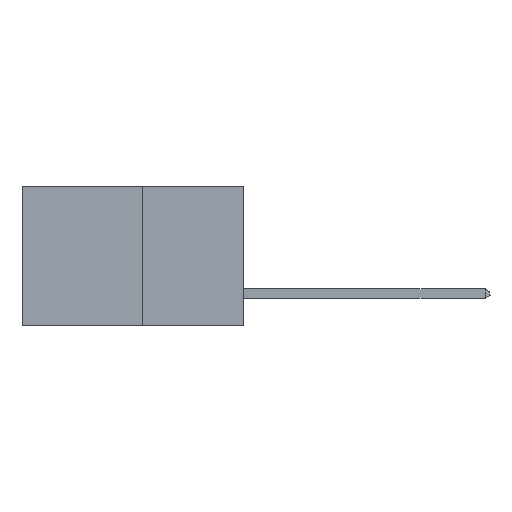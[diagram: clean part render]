
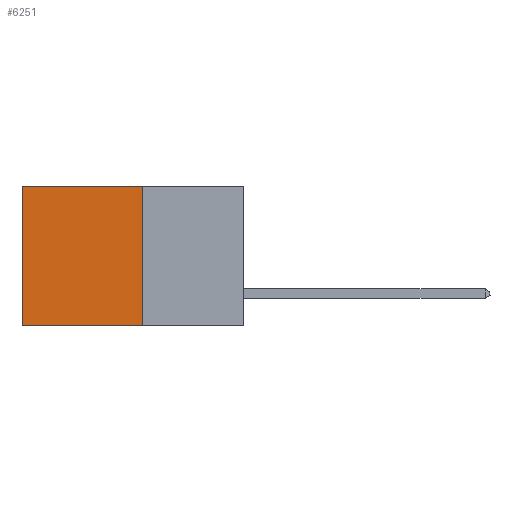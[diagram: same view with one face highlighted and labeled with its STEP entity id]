
A CAD part, left-side view. The second image highlights one B-rep face of the part: STEP entity #6251.
In plain terms, the highlighted planar face has unit normal (-1, 0, 0).
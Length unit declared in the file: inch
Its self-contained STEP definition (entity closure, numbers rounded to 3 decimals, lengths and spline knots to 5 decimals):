
#93 = DIRECTION ( 'NONE',  ( 0., 1., 0. ) ) ;
#866 = ORIENTED_EDGE ( 'NONE', *, *, #18829, .F. ) ;
#1101 = VECTOR ( 'NONE', #10867, 39.37008 ) ;
#3000 = VERTEX_POINT ( 'NONE', #3558 ) ;
#3157 = EDGE_LOOP ( 'NONE', ( #5899, #14427, #866, #17356 ) ) ;
#3518 = PLANE ( 'NONE',  #13369 ) ;
#3558 = CARTESIAN_POINT ( 'NONE',  ( 0.277, 0.27, -0.37 ) ) ;
#3982 = VERTEX_POINT ( 'NONE', #17355 ) ;
#4622 = CARTESIAN_POINT ( 'NONE',  ( 0.277, 0.27, -0.37 ) ) ;
#4717 = LINE ( 'NONE', #21775, #10066 ) ;
#5388 = DIRECTION ( 'NONE',  ( 0., 0., -1. ) ) ;
#5899 = ORIENTED_EDGE ( 'NONE', *, *, #15064, .T. ) ;
#6251 = ADVANCED_FACE ( 'NONE', ( #22441 ), #3518, .F. ) ;
#6295 = CARTESIAN_POINT ( 'NONE',  ( 0.277, 0.59, -0.37 ) ) ;
#6453 = DIRECTION ( 'NONE',  ( 0., 0., -1. ) ) ;
#7672 = EDGE_CURVE ( 'NONE', #15883, #13546, #4717, .T. ) ;
#8906 = CARTESIAN_POINT ( 'NONE',  ( 0.277, 0.27, -0.37 ) ) ;
#10066 = VECTOR ( 'NONE', #93, 39.37008 ) ;
#10346 = EDGE_CURVE ( 'NONE', #3000, #3982, #15606, .T. ) ;
#10867 = DIRECTION ( 'NONE',  ( 0., 1., 0. ) ) ;
#13259 = VECTOR ( 'NONE', #6453, 39.37008 ) ;
#13369 = AXIS2_PLACEMENT_3D ( 'NONE', #8906, #16170, #5388 ) ;
#13546 = VERTEX_POINT ( 'NONE', #20531 ) ;
#14427 = ORIENTED_EDGE ( 'NONE', *, *, #10346, .F. ) ;
#15064 = EDGE_CURVE ( 'NONE', #13546, #3982, #19336, .T. ) ;
#15606 = LINE ( 'NONE', #23340, #1101 ) ;
#15883 = VERTEX_POINT ( 'NONE', #23060 ) ;
#16170 = DIRECTION ( 'NONE',  ( 1., 0., 0. ) ) ;
#17355 = CARTESIAN_POINT ( 'NONE',  ( 0.277, 0.59, -0.37 ) ) ;
#17356 = ORIENTED_EDGE ( 'NONE', *, *, #7672, .T. ) ;
#17961 = VECTOR ( 'NONE', #20644, 39.37008 ) ;
#18829 = EDGE_CURVE ( 'NONE', #15883, #3000, #22703, .T. ) ;
#19336 = LINE ( 'NONE', #6295, #17961 ) ;
#20531 = CARTESIAN_POINT ( 'NONE',  ( 0.277, 0.59, 0. ) ) ;
#20644 = DIRECTION ( 'NONE',  ( 0., 0., -1. ) ) ;
#21775 = CARTESIAN_POINT ( 'NONE',  ( 0.277, 0.27, 0. ) ) ;
#22441 = FACE_OUTER_BOUND ( 'NONE', #3157, .T. ) ;
#22703 = LINE ( 'NONE', #4622, #13259 ) ;
#23060 = CARTESIAN_POINT ( 'NONE',  ( 0.277, 0.27, 0. ) ) ;
#23340 = CARTESIAN_POINT ( 'NONE',  ( 0.277, 0.27, -0.37 ) ) ;
